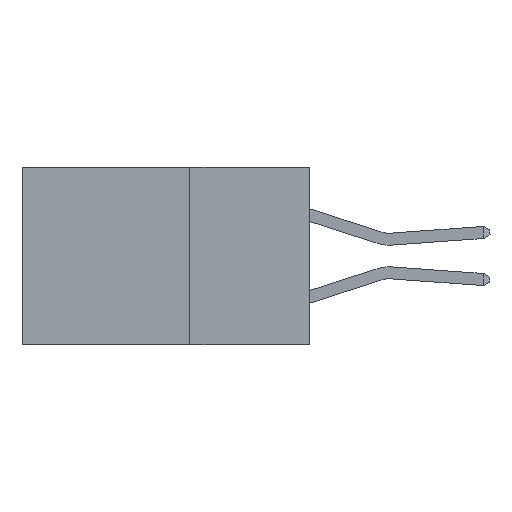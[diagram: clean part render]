
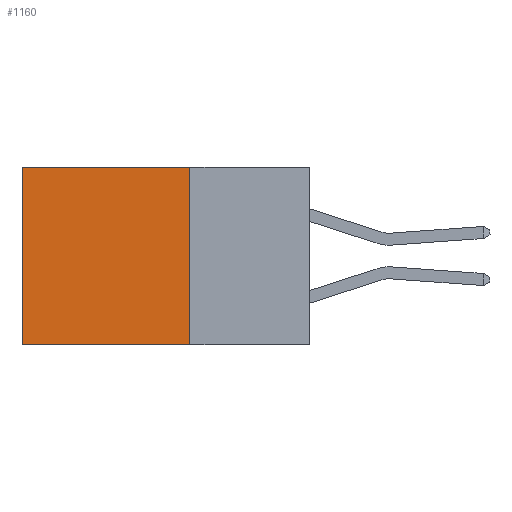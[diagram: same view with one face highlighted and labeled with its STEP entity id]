
A CAD part, left-side view. The second image highlights one B-rep face of the part: STEP entity #1160.
In plain terms, the highlighted planar face has unit normal (-1, 0, 0).
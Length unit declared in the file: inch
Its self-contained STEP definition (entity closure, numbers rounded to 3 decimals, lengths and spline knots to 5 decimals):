
#332 = LINE ( 'NONE', #11497, #9833 ) ;
#459 = DIRECTION ( 'NONE',  ( 0., 0., -1. ) ) ;
#462 = LINE ( 'NONE', #8348, #1070 ) ;
#924 = AXIS2_PLACEMENT_3D ( 'NONE', #11811, #8730, #8728 ) ;
#1070 = VECTOR ( 'NONE', #8333, 39.37008 ) ;
#1160 = ADVANCED_FACE ( 'NONE', ( #4912 ), #8760, .F. ) ;
#1589 = ORIENTED_EDGE ( 'NONE', *, *, #5299, .F. ) ;
#1671 = EDGE_CURVE ( 'NONE', #8912, #3441, #2706, .T. ) ;
#2320 = CARTESIAN_POINT ( 'NONE',  ( 0.298, 0.6, 0. ) ) ;
#2706 = LINE ( 'NONE', #9299, #4597 ) ;
#3047 = VERTEX_POINT ( 'NONE', #10996 ) ;
#3441 = VERTEX_POINT ( 'NONE', #9704 ) ;
#4291 = LINE ( 'NONE', #2320, #11021 ) ;
#4296 = EDGE_CURVE ( 'NONE', #5046, #3047, #4291, .T. ) ;
#4597 = VECTOR ( 'NONE', #10931, 39.37008 ) ;
#4912 = FACE_OUTER_BOUND ( 'NONE', #6655, .T. ) ;
#5046 = VERTEX_POINT ( 'NONE', #8419 ) ;
#5180 = CARTESIAN_POINT ( 'NONE',  ( 0.298, 0.25, 0. ) ) ;
#5238 = ORIENTED_EDGE ( 'NONE', *, *, #4296, .T. ) ;
#5299 = EDGE_CURVE ( 'NONE', #3441, #3047, #332, .T. ) ;
#6109 = ORIENTED_EDGE ( 'NONE', *, *, #1671, .F. ) ;
#6140 = EDGE_CURVE ( 'NONE', #8912, #5046, #462, .T. ) ;
#6655 = EDGE_LOOP ( 'NONE', ( #5238, #1589, #6109, #9486 ) ) ;
#8333 = DIRECTION ( 'NONE',  ( 0., 1., 0. ) ) ;
#8348 = CARTESIAN_POINT ( 'NONE',  ( 0.298, 0.25, 0. ) ) ;
#8419 = CARTESIAN_POINT ( 'NONE',  ( 0.298, 0.6, 0. ) ) ;
#8728 = DIRECTION ( 'NONE',  ( 0., 0., -1. ) ) ;
#8730 = DIRECTION ( 'NONE',  ( 1., 0., 0. ) ) ;
#8760 = PLANE ( 'NONE',  #924 ) ;
#8912 = VERTEX_POINT ( 'NONE', #5180 ) ;
#9299 = CARTESIAN_POINT ( 'NONE',  ( 0.298, 0.25, 0. ) ) ;
#9486 = ORIENTED_EDGE ( 'NONE', *, *, #6140, .T. ) ;
#9704 = CARTESIAN_POINT ( 'NONE',  ( 0.298, 0.25, -0.37 ) ) ;
#9833 = VECTOR ( 'NONE', #11015, 39.37008 ) ;
#10931 = DIRECTION ( 'NONE',  ( 0., 0., -1. ) ) ;
#10996 = CARTESIAN_POINT ( 'NONE',  ( 0.298, 0.6, -0.37 ) ) ;
#11015 = DIRECTION ( 'NONE',  ( 0., 1., 0. ) ) ;
#11021 = VECTOR ( 'NONE', #459, 39.37008 ) ;
#11497 = CARTESIAN_POINT ( 'NONE',  ( 0.298, 0.25, -0.37 ) ) ;
#11811 = CARTESIAN_POINT ( 'NONE',  ( 0.298, 0.25, 0. ) ) ;
